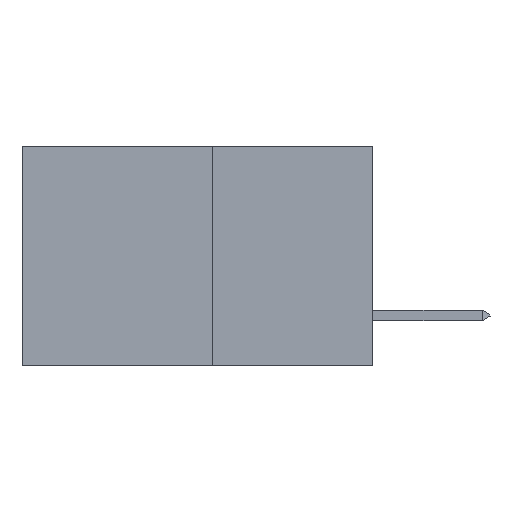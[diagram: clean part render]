
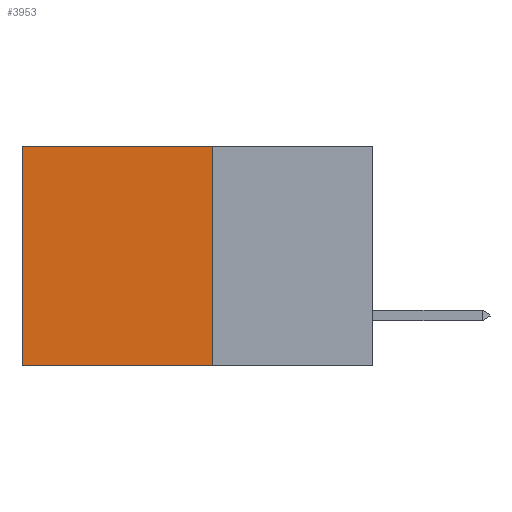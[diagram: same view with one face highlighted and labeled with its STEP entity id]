
A CAD part, left-side view. The second image highlights one B-rep face of the part: STEP entity #3953.
In plain terms, the highlighted planar face has unit normal (-1, 0, 0).
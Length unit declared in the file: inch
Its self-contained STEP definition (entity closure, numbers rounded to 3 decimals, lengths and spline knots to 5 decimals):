
#309 = LINE ( 'NONE', #11158, #26289 ) ;
#1017 = DIRECTION ( 'NONE',  ( 0., 0., -1. ) ) ;
#1470 = CARTESIAN_POINT ( 'NONE',  ( 0.277, 0.27, 0. ) ) ;
#3761 = CARTESIAN_POINT ( 'NONE',  ( 0.277, 0.59, 0. ) ) ;
#3953 = ADVANCED_FACE ( 'NONE', ( #11097 ), #25338, .F. ) ;
#4409 = CARTESIAN_POINT ( 'NONE',  ( 0.277, 0.27, 0. ) ) ;
#5373 = ORIENTED_EDGE ( 'NONE', *, *, #25952, .T. ) ;
#7658 = EDGE_LOOP ( 'NONE', ( #13159, #11072, #30092, #5373 ) ) ;
#7686 = VERTEX_POINT ( 'NONE', #9327 ) ;
#7721 = EDGE_CURVE ( 'NONE', #23516, #7686, #9289, .T. ) ;
#7989 = VECTOR ( 'NONE', #21249, 39.37008 ) ;
#8637 = DIRECTION ( 'NONE',  ( 0., 1., 0. ) ) ;
#8704 = CARTESIAN_POINT ( 'NONE',  ( 0.277, 0.27, -0.37 ) ) ;
#9289 = LINE ( 'NONE', #9359, #21843 ) ;
#9327 = CARTESIAN_POINT ( 'NONE',  ( 0.277, 0.59, -0.37 ) ) ;
#9359 = CARTESIAN_POINT ( 'NONE',  ( 0.277, 0.27, -0.37 ) ) ;
#11072 = ORIENTED_EDGE ( 'NONE', *, *, #7721, .F. ) ;
#11097 = FACE_OUTER_BOUND ( 'NONE', #7658, .T. ) ;
#11158 = CARTESIAN_POINT ( 'NONE',  ( 0.277, 0.59, -0.37 ) ) ;
#13010 = CARTESIAN_POINT ( 'NONE',  ( 0.277, 0.27, -0.37 ) ) ;
#13159 = ORIENTED_EDGE ( 'NONE', *, *, #14513, .T. ) ;
#13810 = DIRECTION ( 'NONE',  ( 0., 0., -1. ) ) ;
#14278 = DIRECTION ( 'NONE',  ( 1., 0., 0. ) ) ;
#14513 = EDGE_CURVE ( 'NONE', #25809, #7686, #309, .T. ) ;
#17792 = AXIS2_PLACEMENT_3D ( 'NONE', #25304, #14278, #13810 ) ;
#18788 = VECTOR ( 'NONE', #24545, 39.37008 ) ;
#19857 = EDGE_CURVE ( 'NONE', #32354, #23516, #21411, .T. ) ;
#21249 = DIRECTION ( 'NONE',  ( 0., 0., -1. ) ) ;
#21411 = LINE ( 'NONE', #8704, #7989 ) ;
#21843 = VECTOR ( 'NONE', #8637, 39.37008 ) ;
#23516 = VERTEX_POINT ( 'NONE', #13010 ) ;
#24545 = DIRECTION ( 'NONE',  ( 0., 1., 0. ) ) ;
#25304 = CARTESIAN_POINT ( 'NONE',  ( 0.277, 0.27, -0.37 ) ) ;
#25338 = PLANE ( 'NONE',  #17792 ) ;
#25809 = VERTEX_POINT ( 'NONE', #3761 ) ;
#25952 = EDGE_CURVE ( 'NONE', #32354, #25809, #31055, .T. ) ;
#26289 = VECTOR ( 'NONE', #1017, 39.37008 ) ;
#30092 = ORIENTED_EDGE ( 'NONE', *, *, #19857, .F. ) ;
#31055 = LINE ( 'NONE', #4409, #18788 ) ;
#32354 = VERTEX_POINT ( 'NONE', #1470 ) ;
